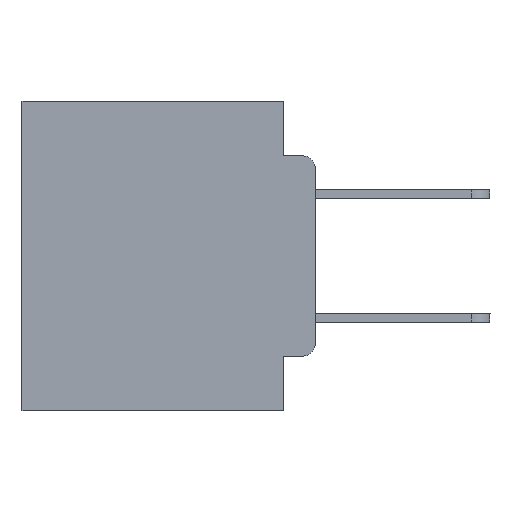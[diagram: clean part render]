
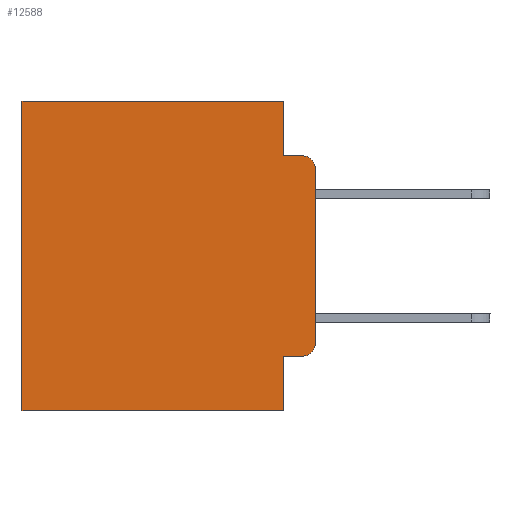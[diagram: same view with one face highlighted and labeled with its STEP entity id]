
A CAD part, left-side view. The second image highlights one B-rep face of the part: STEP entity #12588.
In plain terms, the highlighted planar face has unit normal (-1, 0, 0).
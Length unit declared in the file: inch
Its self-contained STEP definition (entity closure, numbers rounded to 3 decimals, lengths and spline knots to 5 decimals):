
#101 = CARTESIAN_POINT ( 'NONE',  ( 0.298, 0.051, 0. ) ) ;
#111 = ORIENTED_EDGE ( 'NONE', *, *, #17628, .T. ) ;
#155 = PLANE ( 'NONE',  #9811 ) ;
#418 = CARTESIAN_POINT ( 'NONE',  ( 0.298, 0.051, -0.4115 ) ) ;
#564 = CARTESIAN_POINT ( 'NONE',  ( 0.298, 0.473, -0.5 ) ) ;
#994 = EDGE_LOOP ( 'NONE', ( #27290, #19303, #23501, #13217, #3921, #11313, #16492, #1311, #10958, #111 ) ) ;
#1311 = ORIENTED_EDGE ( 'NONE', *, *, #22428, .F. ) ;
#1458 = DIRECTION ( 'NONE',  ( 0., 0., -1. ) ) ;
#1992 = LINE ( 'NONE', #23533, #27588 ) ;
#2221 = DIRECTION ( 'NONE',  ( 1., 0., 0. ) ) ;
#2672 = CIRCLE ( 'NONE', #8062, 0.02 ) ;
#3263 = VERTEX_POINT ( 'NONE', #22280 ) ;
#3694 = EDGE_CURVE ( 'NONE', #21977, #7809, #15819, .T. ) ;
#3921 = ORIENTED_EDGE ( 'NONE', *, *, #20678, .T. ) ;
#4131 = DIRECTION ( 'NONE',  ( 0., 0., -1. ) ) ;
#4199 = LINE ( 'NONE', #12537, #13597 ) ;
#4361 = CARTESIAN_POINT ( 'NONE',  ( 0.298, 0.051, -0.0885 ) ) ;
#4992 = CARTESIAN_POINT ( 'NONE',  ( 0.298, 0.02, -0.1085 ) ) ;
#5688 = LINE ( 'NONE', #18956, #10045 ) ;
#5950 = CARTESIAN_POINT ( 'NONE',  ( 0.298, 0.02, -0.3915 ) ) ;
#6238 = DIRECTION ( 'NONE',  ( 0., 0., -1. ) ) ;
#6685 = DIRECTION ( 'NONE',  ( 0., 1., 0. ) ) ;
#7138 = DIRECTION ( 'NONE',  ( 0., 0., -1. ) ) ;
#7285 = DIRECTION ( 'NONE',  ( 0., 1., 0. ) ) ;
#7809 = VERTEX_POINT ( 'NONE', #8460 ) ;
#7835 = VECTOR ( 'NONE', #7285, 39.37008 ) ;
#8062 = AXIS2_PLACEMENT_3D ( 'NONE', #5950, #20736, #27120 ) ;
#8167 = LINE ( 'NONE', #4361, #14212 ) ;
#8197 = LINE ( 'NONE', #22616, #17279 ) ;
#8250 = DIRECTION ( 'NONE',  ( 0., -1., 0. ) ) ;
#8460 = CARTESIAN_POINT ( 'NONE',  ( 0.298, 0.02, -0.4115 ) ) ;
#9751 = DIRECTION ( 'NONE',  ( 0., 0., -1. ) ) ;
#9811 = AXIS2_PLACEMENT_3D ( 'NONE', #14938, #2221, #4131 ) ;
#10045 = VECTOR ( 'NONE', #19323, 39.37008 ) ;
#10958 = ORIENTED_EDGE ( 'NONE', *, *, #3694, .T. ) ;
#11019 = DIRECTION ( 'NONE',  ( 0., -1., 0. ) ) ;
#11313 = ORIENTED_EDGE ( 'NONE', *, *, #25994, .T. ) ;
#12537 = CARTESIAN_POINT ( 'NONE',  ( 0.298, 0.051, 0. ) ) ;
#12588 = ADVANCED_FACE ( 'NONE', ( #15725 ), #155, .F. ) ;
#12877 = EDGE_CURVE ( 'NONE', #23269, #24539, #27152, .T. ) ;
#13217 = ORIENTED_EDGE ( 'NONE', *, *, #26126, .F. ) ;
#13408 = CARTESIAN_POINT ( 'NONE',  ( 0.298, 0.02, -0.0885 ) ) ;
#13597 = VECTOR ( 'NONE', #1458, 39.37008 ) ;
#13873 = VERTEX_POINT ( 'NONE', #564 ) ;
#14212 = VECTOR ( 'NONE', #11019, 39.37008 ) ;
#14648 = CARTESIAN_POINT ( 'NONE',  ( 0.298, 0.051, -0.0885 ) ) ;
#14938 = CARTESIAN_POINT ( 'NONE',  ( 0.298, 0., 0. ) ) ;
#15550 = CARTESIAN_POINT ( 'NONE',  ( 0.298, 0.473, 0. ) ) ;
#15725 = FACE_OUTER_BOUND ( 'NONE', #994, .T. ) ;
#15819 = LINE ( 'NONE', #19064, #17837 ) ;
#16222 = VERTEX_POINT ( 'NONE', #14648 ) ;
#16492 = ORIENTED_EDGE ( 'NONE', *, *, #22510, .F. ) ;
#16751 = VERTEX_POINT ( 'NONE', #15550 ) ;
#17279 = VECTOR ( 'NONE', #9751, 39.37008 ) ;
#17459 = LINE ( 'NONE', #25140, #21874 ) ;
#17628 = EDGE_CURVE ( 'NONE', #7809, #3263, #2672, .T. ) ;
#17837 = VECTOR ( 'NONE', #8250, 39.37008 ) ;
#17855 = DIRECTION ( 'NONE',  ( -1., 0., 0. ) ) ;
#18382 = CARTESIAN_POINT ( 'NONE',  ( 0.298, 0., 0. ) ) ;
#18956 = CARTESIAN_POINT ( 'NONE',  ( 0.298, 0., 0. ) ) ;
#19064 = CARTESIAN_POINT ( 'NONE',  ( 0.298, 0.051, -0.4115 ) ) ;
#19303 = ORIENTED_EDGE ( 'NONE', *, *, #12877, .T. ) ;
#19323 = DIRECTION ( 'NONE',  ( 0., 0., -1. ) ) ;
#19353 = CARTESIAN_POINT ( 'NONE',  ( 0.298, 0., -0.1085 ) ) ;
#20666 = LINE ( 'NONE', #18382, #7835 ) ;
#20678 = EDGE_CURVE ( 'NONE', #25017, #16751, #20666, .T. ) ;
#20736 = DIRECTION ( 'NONE',  ( -1., 0., 0. ) ) ;
#21007 = EDGE_CURVE ( 'NONE', #16222, #24539, #8167, .T. ) ;
#21874 = VECTOR ( 'NONE', #6238, 39.37008 ) ;
#21977 = VERTEX_POINT ( 'NONE', #418 ) ;
#22280 = CARTESIAN_POINT ( 'NONE',  ( 0.298, 0., -0.3915 ) ) ;
#22428 = EDGE_CURVE ( 'NONE', #21977, #23162, #17459, .T. ) ;
#22510 = EDGE_CURVE ( 'NONE', #23162, #13873, #1992, .T. ) ;
#22616 = CARTESIAN_POINT ( 'NONE',  ( 0.298, 0.473, 0. ) ) ;
#22928 = AXIS2_PLACEMENT_3D ( 'NONE', #4992, #17855, #7138 ) ;
#23162 = VERTEX_POINT ( 'NONE', #26118 ) ;
#23269 = VERTEX_POINT ( 'NONE', #19353 ) ;
#23501 = ORIENTED_EDGE ( 'NONE', *, *, #21007, .F. ) ;
#23533 = CARTESIAN_POINT ( 'NONE',  ( 0.298, 0., -0.5 ) ) ;
#23778 = EDGE_CURVE ( 'NONE', #23269, #3263, #5688, .T. ) ;
#24539 = VERTEX_POINT ( 'NONE', #13408 ) ;
#25017 = VERTEX_POINT ( 'NONE', #101 ) ;
#25140 = CARTESIAN_POINT ( 'NONE',  ( 0.298, 0.051, 0. ) ) ;
#25994 = EDGE_CURVE ( 'NONE', #16751, #13873, #8197, .T. ) ;
#26118 = CARTESIAN_POINT ( 'NONE',  ( 0.298, 0.051, -0.5 ) ) ;
#26126 = EDGE_CURVE ( 'NONE', #25017, #16222, #4199, .T. ) ;
#27120 = DIRECTION ( 'NONE',  ( 0., 0., -1. ) ) ;
#27152 = CIRCLE ( 'NONE', #22928, 0.02 ) ;
#27290 = ORIENTED_EDGE ( 'NONE', *, *, #23778, .F. ) ;
#27588 = VECTOR ( 'NONE', #6685, 39.37008 ) ;
